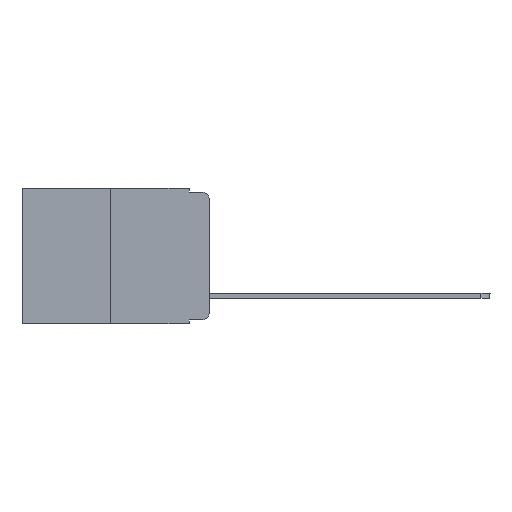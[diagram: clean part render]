
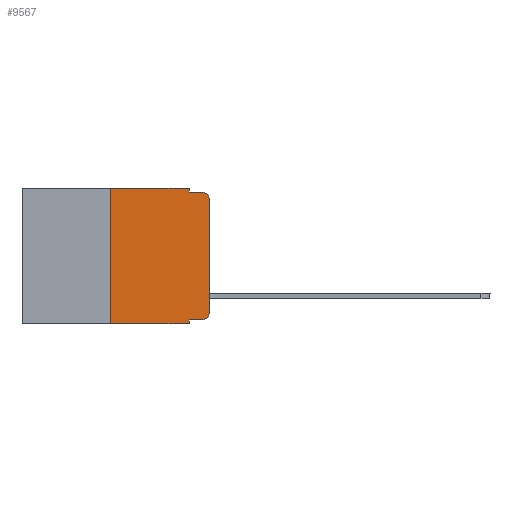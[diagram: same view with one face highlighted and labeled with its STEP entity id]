
A CAD part, left-side view. The second image highlights one B-rep face of the part: STEP entity #9567.
In plain terms, the highlighted planar face has unit normal (-1, 0, 0).
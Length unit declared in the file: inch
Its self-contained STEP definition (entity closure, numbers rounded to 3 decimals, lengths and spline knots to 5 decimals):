
#281 = DIRECTION ( 'NONE',  ( 0., 0., 1. ) ) ;
#295 = CARTESIAN_POINT ( 'NONE',  ( 0., 0., -0.03 ) ) ;
#310 = ORIENTED_EDGE ( 'NONE', *, *, #10799, .T. ) ;
#696 = CARTESIAN_POINT ( 'NONE',  ( 0., 0.25, 0. ) ) ;
#789 = CARTESIAN_POINT ( 'NONE',  ( 0., 0.473, 0. ) ) ;
#844 = EDGE_CURVE ( 'NONE', #8385, #11290, #5274, .T. ) ;
#1473 = VERTEX_POINT ( 'NONE', #2445 ) ;
#1688 = FACE_OUTER_BOUND ( 'NONE', #4122, .T. ) ;
#2010 = CARTESIAN_POINT ( 'NONE',  ( 0., 0.051, 0. ) ) ;
#2073 = CARTESIAN_POINT ( 'NONE',  ( 0., 0., 0. ) ) ;
#2107 = CARTESIAN_POINT ( 'NONE',  ( 0., 0.02, -0.03 ) ) ;
#2180 = DIRECTION ( 'NONE',  ( 0., -1., 0. ) ) ;
#2236 = CARTESIAN_POINT ( 'NONE',  ( 0., 0.051, 0. ) ) ;
#2323 = LINE ( 'NONE', #5893, #10677 ) ;
#2328 = CARTESIAN_POINT ( 'NONE',  ( 0., 0.051, -0.01 ) ) ;
#2445 = CARTESIAN_POINT ( 'NONE',  ( 0., 0.051, -0.343 ) ) ;
#2724 = EDGE_CURVE ( 'NONE', #10986, #11290, #2323, .T. ) ;
#3520 = DIRECTION ( 'NONE',  ( 0., 0., -1. ) ) ;
#3533 = ORIENTED_EDGE ( 'NONE', *, *, #5766, .F. ) ;
#3603 = EDGE_CURVE ( 'NONE', #4013, #11682, #7698, .T. ) ;
#3652 = CARTESIAN_POINT ( 'NONE',  ( 0., 0., -0.313 ) ) ;
#3837 = ORIENTED_EDGE ( 'NONE', *, *, #844, .T. ) ;
#3876 = ORIENTED_EDGE ( 'NONE', *, *, #3603, .T. ) ;
#4013 = VERTEX_POINT ( 'NONE', #8639 ) ;
#4095 = ORIENTED_EDGE ( 'NONE', *, *, #10521, .F. ) ;
#4122 = EDGE_LOOP ( 'NONE', ( #5603, #3837, #5405, #9938, #11593, #3533, #310, #4095, #4977, #3876 ) ) ;
#4151 = DIRECTION ( 'NONE',  ( 0., 0., 1. ) ) ;
#4296 = DIRECTION ( 'NONE',  ( 0., 0., -1. ) ) ;
#4344 = VECTOR ( 'NONE', #8487, 39.37008 ) ;
#4457 = EDGE_CURVE ( 'NONE', #6986, #5470, #6602, .T. ) ;
#4554 = LINE ( 'NONE', #11060, #5313 ) ;
#4697 = DIRECTION ( 'NONE',  ( 0., 0., -1. ) ) ;
#4977 = ORIENTED_EDGE ( 'NONE', *, *, #9161, .T. ) ;
#5064 = VECTOR ( 'NONE', #4151, 39.37008 ) ;
#5148 = VECTOR ( 'NONE', #8746, 39.37008 ) ;
#5238 = LINE ( 'NONE', #696, #5064 ) ;
#5274 = CIRCLE ( 'NONE', #10581, 0.02 ) ;
#5313 = VECTOR ( 'NONE', #10090, 39.37008 ) ;
#5328 = PLANE ( 'NONE',  #8149 ) ;
#5405 = ORIENTED_EDGE ( 'NONE', *, *, #2724, .F. ) ;
#5470 = VERTEX_POINT ( 'NONE', #5530 ) ;
#5530 = CARTESIAN_POINT ( 'NONE',  ( 0., 0.051, 0. ) ) ;
#5538 = CARTESIAN_POINT ( 'NONE',  ( 0., 0.02, -0.01 ) ) ;
#5603 = ORIENTED_EDGE ( 'NONE', *, *, #8781, .T. ) ;
#5623 = EDGE_CURVE ( 'NONE', #5470, #10986, #6717, .T. ) ;
#5766 = EDGE_CURVE ( 'NONE', #7530, #6986, #5238, .T. ) ;
#5893 = CARTESIAN_POINT ( 'NONE',  ( 0., 0.051, -0.01 ) ) ;
#6121 = CARTESIAN_POINT ( 'NONE',  ( 0., 0.25, 0. ) ) ;
#6195 = CARTESIAN_POINT ( 'NONE',  ( 0., 0.02, -0.313 ) ) ;
#6351 = AXIS2_PLACEMENT_3D ( 'NONE', #6195, #9777, #4296 ) ;
#6602 = LINE ( 'NONE', #9284, #9029 ) ;
#6717 = LINE ( 'NONE', #2010, #11348 ) ;
#6798 = DIRECTION ( 'NONE',  ( 0., -1., 0. ) ) ;
#6833 = LINE ( 'NONE', #2236, #5148 ) ;
#6986 = VERTEX_POINT ( 'NONE', #6121 ) ;
#7530 = VERTEX_POINT ( 'NONE', #9427 ) ;
#7698 = CIRCLE ( 'NONE', #6351, 0.02 ) ;
#7876 = VECTOR ( 'NONE', #281, 39.37008 ) ;
#8149 = AXIS2_PLACEMENT_3D ( 'NONE', #789, #11680, #3520 ) ;
#8385 = VERTEX_POINT ( 'NONE', #295 ) ;
#8487 = DIRECTION ( 'NONE',  ( 0., -1., 0. ) ) ;
#8639 = CARTESIAN_POINT ( 'NONE',  ( 0., 0.02, -0.333 ) ) ;
#8746 = DIRECTION ( 'NONE',  ( 0., 0., -1. ) ) ;
#8781 = EDGE_CURVE ( 'NONE', #11682, #8385, #10110, .T. ) ;
#9029 = VECTOR ( 'NONE', #2180, 39.37008 ) ;
#9153 = CARTESIAN_POINT ( 'NONE',  ( 0., 0.051, -0.333 ) ) ;
#9161 = EDGE_CURVE ( 'NONE', #10875, #4013, #10142, .T. ) ;
#9284 = CARTESIAN_POINT ( 'NONE',  ( 0., 0.473, 0. ) ) ;
#9376 = DIRECTION ( 'NONE',  ( -1., 0., 0. ) ) ;
#9427 = CARTESIAN_POINT ( 'NONE',  ( 0., 0.25, -0.343 ) ) ;
#9567 = ADVANCED_FACE ( 'NONE', ( #1688 ), #5328, .F. ) ;
#9777 = DIRECTION ( 'NONE',  ( -1., 0., 0. ) ) ;
#9938 = ORIENTED_EDGE ( 'NONE', *, *, #5623, .F. ) ;
#10090 = DIRECTION ( 'NONE',  ( 0., -1., 0. ) ) ;
#10110 = LINE ( 'NONE', #2073, #7876 ) ;
#10142 = LINE ( 'NONE', #11286, #4344 ) ;
#10521 = EDGE_CURVE ( 'NONE', #10875, #1473, #6833, .T. ) ;
#10581 = AXIS2_PLACEMENT_3D ( 'NONE', #2107, #9376, #11052 ) ;
#10677 = VECTOR ( 'NONE', #6798, 39.37008 ) ;
#10799 = EDGE_CURVE ( 'NONE', #7530, #1473, #4554, .T. ) ;
#10875 = VERTEX_POINT ( 'NONE', #9153 ) ;
#10986 = VERTEX_POINT ( 'NONE', #2328 ) ;
#11052 = DIRECTION ( 'NONE',  ( 0., 0., -1. ) ) ;
#11060 = CARTESIAN_POINT ( 'NONE',  ( 0., 0.473, -0.343 ) ) ;
#11286 = CARTESIAN_POINT ( 'NONE',  ( 0., 0.051, -0.333 ) ) ;
#11290 = VERTEX_POINT ( 'NONE', #5538 ) ;
#11348 = VECTOR ( 'NONE', #4697, 39.37008 ) ;
#11593 = ORIENTED_EDGE ( 'NONE', *, *, #4457, .F. ) ;
#11680 = DIRECTION ( 'NONE',  ( 1., 0., 0. ) ) ;
#11682 = VERTEX_POINT ( 'NONE', #3652 ) ;
